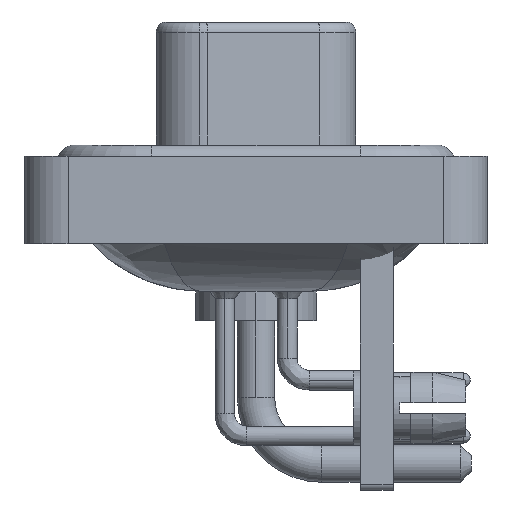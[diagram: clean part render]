
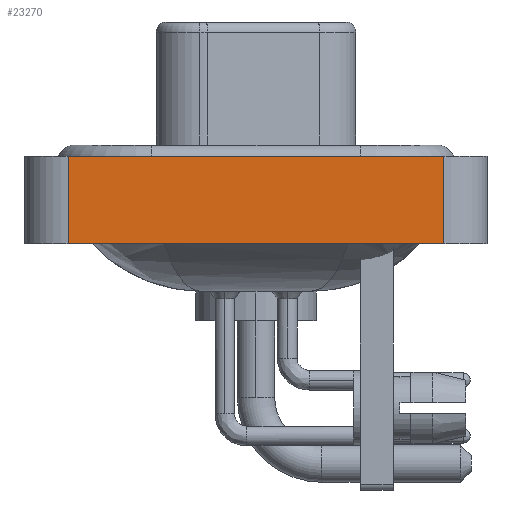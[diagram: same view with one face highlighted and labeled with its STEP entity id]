
A CAD part, left-side view. The second image highlights one B-rep face of the part: STEP entity #23270.
In plain terms, the highlighted planar face has unit normal (-1, 0, 0).
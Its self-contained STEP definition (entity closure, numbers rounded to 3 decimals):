
#883 = ORIENTED_EDGE ( 'NONE', *, *, #25672, .T. ) ;
#1805 = ORIENTED_EDGE ( 'NONE', *, *, #20470, .F. ) ;
#1907 = DIRECTION ( 'NONE',  ( -1., 0., 0. ) ) ;
#4014 = LINE ( 'NONE', #26647, #16105 ) ;
#4111 = VERTEX_POINT ( 'NONE', #15900 ) ;
#4246 = VECTOR ( 'NONE', #5752, 1000. ) ;
#4332 = DIRECTION ( 'NONE',  ( 0., -1., 0. ) ) ;
#4663 = VECTOR ( 'NONE', #27162, 1000. ) ;
#5321 = CARTESIAN_POINT ( 'NONE',  ( -7.35, -8.55, -3.6 ) ) ;
#5752 = DIRECTION ( 'NONE',  ( 0., -1., 0. ) ) ;
#6931 = ORIENTED_EDGE ( 'NONE', *, *, #14194, .F. ) ;
#8746 = LINE ( 'NONE', #18779, #30783 ) ;
#9509 = FACE_OUTER_BOUND ( 'NONE', #20157, .T. ) ;
#11785 = CARTESIAN_POINT ( 'NONE',  ( -7.35, 8.55, -3.6 ) ) ;
#13208 = CARTESIAN_POINT ( 'NONE',  ( -7.35, -8.55, -3.6 ) ) ;
#13769 = DIRECTION ( 'NONE',  ( 0., 0., 1. ) ) ;
#14194 = EDGE_CURVE ( 'NONE', #23933, #4111, #4014, .T. ) ;
#14213 = CARTESIAN_POINT ( 'NONE',  ( -7.35, -8.55, -3.6 ) ) ;
#14387 = LINE ( 'NONE', #11785, #4663 ) ;
#14559 = EDGE_CURVE ( 'NONE', #19815, #18917, #15472, .T. ) ;
#15472 = LINE ( 'NONE', #13208, #4246 ) ;
#15900 = CARTESIAN_POINT ( 'NONE',  ( -7.35, -8.55, 0.4 ) ) ;
#16105 = VECTOR ( 'NONE', #4332, 1000. ) ;
#18779 = CARTESIAN_POINT ( 'NONE',  ( -7.35, -8.55, -3.6 ) ) ;
#18917 = VERTEX_POINT ( 'NONE', #5321 ) ;
#19058 = PLANE ( 'NONE',  #21268 ) ;
#19815 = VERTEX_POINT ( 'NONE', #20450 ) ;
#20157 = EDGE_LOOP ( 'NONE', ( #883, #6931, #1805, #28719 ) ) ;
#20450 = CARTESIAN_POINT ( 'NONE',  ( -7.35, 8.55, -3.6 ) ) ;
#20470 = EDGE_CURVE ( 'NONE', #19815, #23933, #14387, .T. ) ;
#21268 = AXIS2_PLACEMENT_3D ( 'NONE', #14213, #1907, #31315 ) ;
#23270 = ADVANCED_FACE ( 'NONE', ( #9509 ), #19058, .T. ) ;
#23933 = VERTEX_POINT ( 'NONE', #28417 ) ;
#25672 = EDGE_CURVE ( 'NONE', #18917, #4111, #8746, .T. ) ;
#26647 = CARTESIAN_POINT ( 'NONE',  ( -7.35, -8.55, 0.4 ) ) ;
#27162 = DIRECTION ( 'NONE',  ( 0., 0., 1. ) ) ;
#28417 = CARTESIAN_POINT ( 'NONE',  ( -7.35, 8.55, 0.4 ) ) ;
#28719 = ORIENTED_EDGE ( 'NONE', *, *, #14559, .T. ) ;
#30783 = VECTOR ( 'NONE', #13769, 1000. ) ;
#31315 = DIRECTION ( 'NONE',  ( 0., 0., 1. ) ) ;
